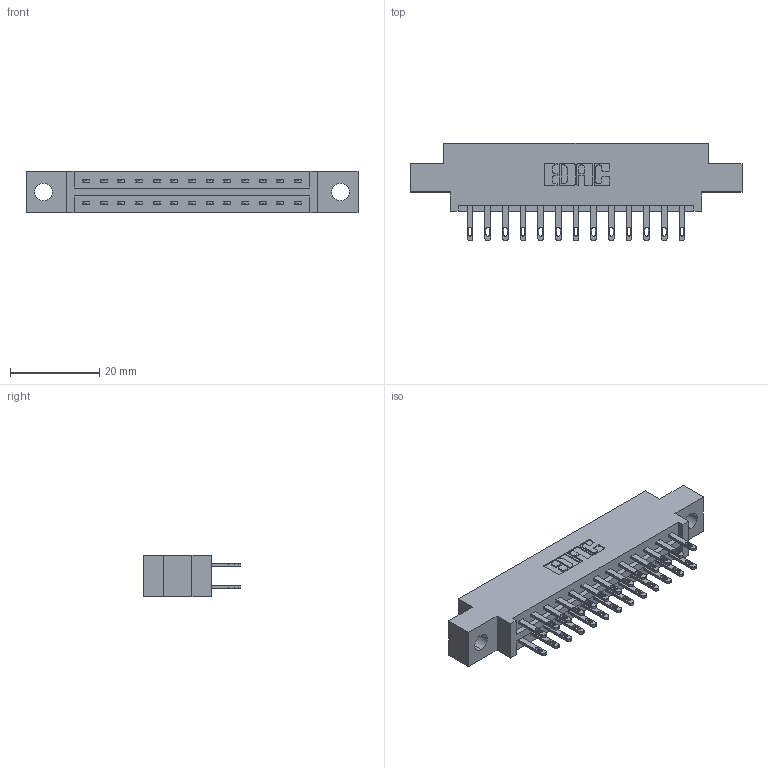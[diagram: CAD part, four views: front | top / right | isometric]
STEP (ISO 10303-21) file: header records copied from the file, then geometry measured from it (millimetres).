
FILE_DESCRIPTION (( 'STEP AP203' ), '1' );
FILE_NAME ('337-026-500-804.STEP', '2019-10-10T21:26:34', ( '' ), ( '' ), 'SwSTEP 2.0', 'SolidWorks 2016', '' );
FILE_SCHEMA (( 'CONFIG_CONTROL_DESIGN' ));
Length unit declared in the file: inch
Products named in the file (3): 337 Part_0.170 Offset - 0.156 Dia-TH; 345-292-001_345-293-100; 337-026-500-804
Assembly tree (27 placements, depth 2):
  337-026-500-804
    337 Part_0.170 Offset - 0.156 Dia-TH
    345-292-001_345-293-100  x26
Bounding box: 74.52 x 21.85 x 9.4 mm (x, y, z)
Volume: 7342 mm3; surface area: 8212.1 mm2
Topology: 27 solids, 27 shells, 1418 faces, 4301 edges, 2866 vertices
Faces by surface type: plane 906, cylinder 512
Entity records: 13895 total; most frequent: CARTESIAN_POINT 2366, ORIENTED_EDGE 2302, DIRECTION 2067, EDGE_CURVE 1151, VECTOR 1019, LINE 1019, VERTEX_POINT 766, AXIS2_PLACEMENT_3D 524
